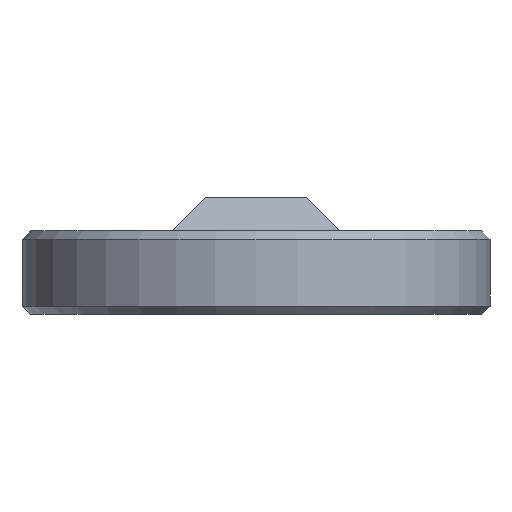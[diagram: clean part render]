
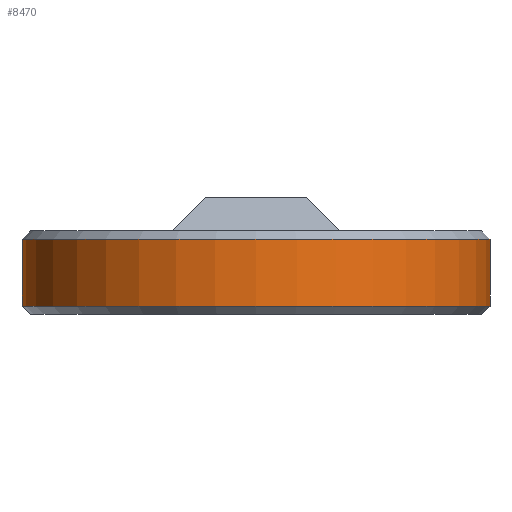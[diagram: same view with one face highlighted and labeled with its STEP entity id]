
A CAD part, left-side view. The second image highlights one B-rep face of the part: STEP entity #8470.
In plain terms, the highlighted cylindrical face has radius 8.89 mm (diameter 17.78 mm), a partial arc.
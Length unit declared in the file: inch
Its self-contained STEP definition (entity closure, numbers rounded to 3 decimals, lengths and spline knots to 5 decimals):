
#154 = VERTEX_POINT ( 'NONE', #10045 ) ;
#240 = DIRECTION ( 'NONE',  ( 0., 0., -1. ) ) ;
#1081 = ORIENTED_EDGE ( 'NONE', *, *, #5029, .T. ) ;
#1156 = CARTESIAN_POINT ( 'NONE',  ( -1.175, 0., 0.0125 ) ) ;
#1710 = AXIS2_PLACEMENT_3D ( 'NONE', #1156, #6815, #10134 ) ;
#1727 = VERTEX_POINT ( 'NONE', #7487 ) ;
#1839 = CARTESIAN_POINT ( 'NONE',  ( -1.175, 0., 0.125 ) ) ;
#2278 = ORIENTED_EDGE ( 'NONE', *, *, #4898, .F. ) ;
#2478 = DIRECTION ( 'NONE',  ( 0., 0., -1. ) ) ;
#2948 = VECTOR ( 'NONE', #2478, 39.37008 ) ;
#3727 = EDGE_CURVE ( 'NONE', #1727, #7293, #9502, .T. ) ;
#4472 = DIRECTION ( 'NONE',  ( 0., 0., -1. ) ) ;
#4618 = ORIENTED_EDGE ( 'NONE', *, *, #8547, .T. ) ;
#4790 = EDGE_LOOP ( 'NONE', ( #7709, #4618, #2278, #1081 ) ) ;
#4898 = EDGE_CURVE ( 'NONE', #8455, #154, #7723, .T. ) ;
#5029 = EDGE_CURVE ( 'NONE', #8455, #1727, #6966, .T. ) ;
#5232 = VECTOR ( 'NONE', #4472, 39.37008 ) ;
#5834 = CARTESIAN_POINT ( 'NONE',  ( -1.175, -0.35, 0.125 ) ) ;
#6770 = CARTESIAN_POINT ( 'NONE',  ( -1.175, 0., 0.1125 ) ) ;
#6815 = DIRECTION ( 'NONE',  ( 0., 0., 1. ) ) ;
#6837 = DIRECTION ( 'NONE',  ( 0., 0., -1. ) ) ;
#6849 = CARTESIAN_POINT ( 'NONE',  ( -1.175, 0.35, 0.125 ) ) ;
#6966 = CIRCLE ( 'NONE', #9125, 0.35 ) ;
#7045 = CARTESIAN_POINT ( 'NONE',  ( -1.175, 0.35, 0.0125 ) ) ;
#7293 = VERTEX_POINT ( 'NONE', #7045 ) ;
#7487 = CARTESIAN_POINT ( 'NONE',  ( -1.175, 0.35, 0.1125 ) ) ;
#7709 = ORIENTED_EDGE ( 'NONE', *, *, #3727, .T. ) ;
#7723 = LINE ( 'NONE', #5834, #2948 ) ;
#8022 = CIRCLE ( 'NONE', #1710, 0.35 ) ;
#8288 = FACE_OUTER_BOUND ( 'NONE', #4790, .T. ) ;
#8455 = VERTEX_POINT ( 'NONE', #9642 ) ;
#8470 = ADVANCED_FACE ( 'NONE', ( #8288 ), #10300, .T. ) ;
#8547 = EDGE_CURVE ( 'NONE', #7293, #154, #8022, .T. ) ;
#8957 = AXIS2_PLACEMENT_3D ( 'NONE', #1839, #240, #9047 ) ;
#9047 = DIRECTION ( 'NONE',  ( 0., -1., 0. ) ) ;
#9125 = AXIS2_PLACEMENT_3D ( 'NONE', #6770, #6837, #9198 ) ;
#9198 = DIRECTION ( 'NONE',  ( 0., 1., 0. ) ) ;
#9502 = LINE ( 'NONE', #6849, #5232 ) ;
#9642 = CARTESIAN_POINT ( 'NONE',  ( -1.175, -0.35, 0.1125 ) ) ;
#10045 = CARTESIAN_POINT ( 'NONE',  ( -1.175, -0.35, 0.0125 ) ) ;
#10134 = DIRECTION ( 'NONE',  ( 0., 1., 0. ) ) ;
#10300 = CYLINDRICAL_SURFACE ( 'NONE', #8957, 0.35 ) ;
